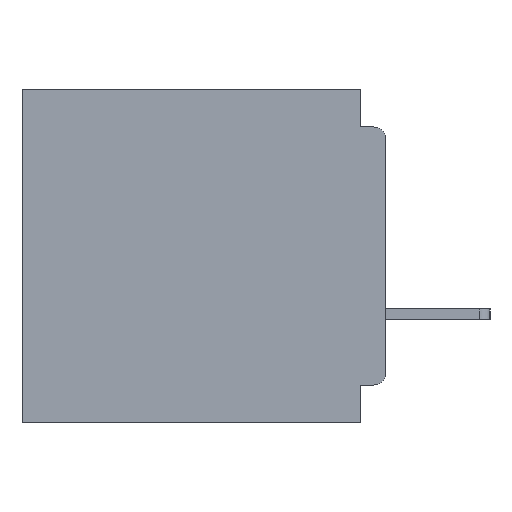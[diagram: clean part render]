
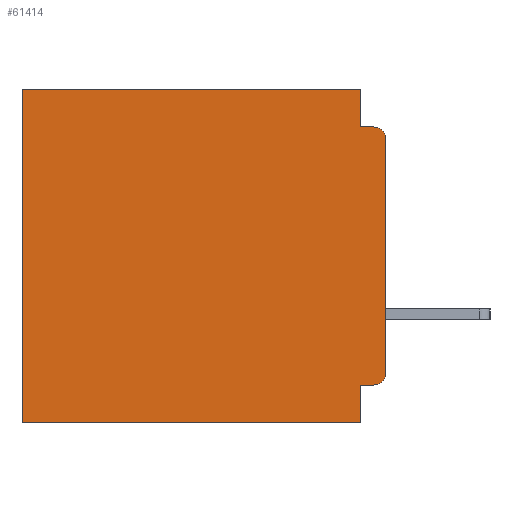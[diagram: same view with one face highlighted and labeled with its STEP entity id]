
A CAD part, left-side view. The second image highlights one B-rep face of the part: STEP entity #61414.
In plain terms, the highlighted planar face has unit normal (-1, 0, 0).
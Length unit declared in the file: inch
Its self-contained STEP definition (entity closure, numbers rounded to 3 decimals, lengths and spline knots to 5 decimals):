
#351 = CARTESIAN_POINT ( 'NONE',  ( 0.3, 0.437, 0. ) ) ;
#916 = ORIENTED_EDGE ( 'NONE', *, *, #24762, .F. ) ;
#1040 = CARTESIAN_POINT ( 'NONE',  ( 0.3, 0.031, -0.355 ) ) ;
#2915 = CARTESIAN_POINT ( 'NONE',  ( 0.3, 0.031, -0.4 ) ) ;
#5442 = CARTESIAN_POINT ( 'NONE',  ( 0.3, 0.015, -0.355 ) ) ;
#6471 = VECTOR ( 'NONE', #7966, 39.37008 ) ;
#6531 = EDGE_CURVE ( 'NONE', #40955, #40975, #32514, .T. ) ;
#6659 = VECTOR ( 'NONE', #20044, 39.37008 ) ;
#7397 = CARTESIAN_POINT ( 'NONE',  ( 0.3, 0., -0.34 ) ) ;
#7966 = DIRECTION ( 'NONE',  ( 0., 0., -1. ) ) ;
#9464 = AXIS2_PLACEMENT_3D ( 'NONE', #40787, #11779, #45653 ) ;
#9572 = DIRECTION ( 'NONE',  ( 0., 0., -1. ) ) ;
#9650 = CARTESIAN_POINT ( 'NONE',  ( 0.3, 0.015, -0.34 ) ) ;
#9901 = VECTOR ( 'NONE', #31762, 39.37008 ) ;
#9990 = VECTOR ( 'NONE', #12274, 39.37008 ) ;
#11779 = DIRECTION ( 'NONE',  ( -1., 0., 0. ) ) ;
#12274 = DIRECTION ( 'NONE',  ( 0., -1., 0. ) ) ;
#12869 = CARTESIAN_POINT ( 'NONE',  ( 0.3, 0.031, -0.4 ) ) ;
#13371 = EDGE_CURVE ( 'NONE', #30575, #21173, #24638, .T. ) ;
#13709 = DIRECTION ( 'NONE',  ( 0., 1., 0. ) ) ;
#13722 = VERTEX_POINT ( 'NONE', #39696 ) ;
#14562 = DIRECTION ( 'NONE',  ( 0., 0., -1. ) ) ;
#14825 = DIRECTION ( 'NONE',  ( 1., 0., 0. ) ) ;
#15060 = EDGE_CURVE ( 'NONE', #29861, #50919, #62801, .T. ) ;
#16568 = ORIENTED_EDGE ( 'NONE', *, *, #6531, .F. ) ;
#17241 = AXIS2_PLACEMENT_3D ( 'NONE', #9650, #43543, #14562 ) ;
#18829 = VECTOR ( 'NONE', #9572, 39.37008 ) ;
#19095 = EDGE_CURVE ( 'NONE', #25048, #40975, #49590, .T. ) ;
#20044 = DIRECTION ( 'NONE',  ( 0., 0., -1. ) ) ;
#20284 = ORIENTED_EDGE ( 'NONE', *, *, #28108, .T. ) ;
#21173 = VERTEX_POINT ( 'NONE', #45372 ) ;
#22085 = CARTESIAN_POINT ( 'NONE',  ( 0.3, 0., 0. ) ) ;
#22993 = LINE ( 'NONE', #50999, #9990 ) ;
#23449 = EDGE_LOOP ( 'NONE', ( #16568, #20284, #916, #38495, #24552, #29394, #49264, #24599, #29490, #45319 ) ) ;
#23520 = CARTESIAN_POINT ( 'NONE',  ( 0.3, 0., -0.355 ) ) ;
#24063 = CARTESIAN_POINT ( 'NONE',  ( 0.3, 0.031, 0. ) ) ;
#24552 = ORIENTED_EDGE ( 'NONE', *, *, #15060, .T. ) ;
#24599 = ORIENTED_EDGE ( 'NONE', *, *, #59962, .F. ) ;
#24638 = LINE ( 'NONE', #34206, #48790 ) ;
#24762 = EDGE_CURVE ( 'NONE', #57571, #13722, #22993, .T. ) ;
#25048 = VERTEX_POINT ( 'NONE', #5442 ) ;
#25126 = CARTESIAN_POINT ( 'NONE',  ( 0.3, 0., -0.4 ) ) ;
#26385 = VECTOR ( 'NONE', #13709, 39.37008 ) ;
#27464 = EDGE_CURVE ( 'NONE', #25048, #47834, #27925, .T. ) ;
#27925 = LINE ( 'NONE', #23520, #26385 ) ;
#28108 = EDGE_CURVE ( 'NONE', #40955, #13722, #39850, .T. ) ;
#29210 = DIRECTION ( 'NONE',  ( 0., 1., 0. ) ) ;
#29394 = ORIENTED_EDGE ( 'NONE', *, *, #47730, .T. ) ;
#29490 = ORIENTED_EDGE ( 'NONE', *, *, #27464, .F. ) ;
#29861 = VERTEX_POINT ( 'NONE', #41222 ) ;
#30575 = VERTEX_POINT ( 'NONE', #2915 ) ;
#31762 = DIRECTION ( 'NONE',  ( 0., 1., 0. ) ) ;
#32514 = LINE ( 'NONE', #25126, #6659 ) ;
#34206 = CARTESIAN_POINT ( 'NONE',  ( 0.3, 0., -0.4 ) ) ;
#35443 = CARTESIAN_POINT ( 'NONE',  ( 0.3, 0.031, -0.045 ) ) ;
#38495 = ORIENTED_EDGE ( 'NONE', *, *, #46556, .F. ) ;
#38903 = PLANE ( 'NONE',  #59714 ) ;
#39696 = CARTESIAN_POINT ( 'NONE',  ( 0.3, 0.015, -0.045 ) ) ;
#39850 = CIRCLE ( 'NONE', #9464, 0.015 ) ;
#40607 = LINE ( 'NONE', #12869, #6471 ) ;
#40787 = CARTESIAN_POINT ( 'NONE',  ( 0.3, 0.015, -0.06 ) ) ;
#40955 = VERTEX_POINT ( 'NONE', #50817 ) ;
#40975 = VERTEX_POINT ( 'NONE', #7397 ) ;
#41222 = CARTESIAN_POINT ( 'NONE',  ( 0.3, 0.031, 0. ) ) ;
#43543 = DIRECTION ( 'NONE',  ( -1., 0., 0. ) ) ;
#43793 = CARTESIAN_POINT ( 'NONE',  ( 0.3, 0., -0.4 ) ) ;
#44497 = LINE ( 'NONE', #24063, #18829 ) ;
#45319 = ORIENTED_EDGE ( 'NONE', *, *, #19095, .T. ) ;
#45372 = CARTESIAN_POINT ( 'NONE',  ( 0.3, 0.437, -0.4 ) ) ;
#45653 = DIRECTION ( 'NONE',  ( 0., 0., -1. ) ) ;
#46224 = FACE_OUTER_BOUND ( 'NONE', #23449, .T. ) ;
#46556 = EDGE_CURVE ( 'NONE', #29861, #57571, #44497, .T. ) ;
#47354 = VECTOR ( 'NONE', #58229, 39.37008 ) ;
#47730 = EDGE_CURVE ( 'NONE', #50919, #21173, #50383, .T. ) ;
#47834 = VERTEX_POINT ( 'NONE', #1040 ) ;
#48657 = DIRECTION ( 'NONE',  ( 0., 0., -1. ) ) ;
#48790 = VECTOR ( 'NONE', #29210, 39.37008 ) ;
#49264 = ORIENTED_EDGE ( 'NONE', *, *, #13371, .F. ) ;
#49590 = CIRCLE ( 'NONE', #17241, 0.015 ) ;
#50383 = LINE ( 'NONE', #53401, #47354 ) ;
#50817 = CARTESIAN_POINT ( 'NONE',  ( 0.3, 0., -0.06 ) ) ;
#50919 = VERTEX_POINT ( 'NONE', #351 ) ;
#50999 = CARTESIAN_POINT ( 'NONE',  ( 0.3, 0., -0.045 ) ) ;
#53401 = CARTESIAN_POINT ( 'NONE',  ( 0.3, 0.437, -0.4 ) ) ;
#57571 = VERTEX_POINT ( 'NONE', #35443 ) ;
#58229 = DIRECTION ( 'NONE',  ( 0., 0., -1. ) ) ;
#59714 = AXIS2_PLACEMENT_3D ( 'NONE', #43793, #14825, #48657 ) ;
#59962 = EDGE_CURVE ( 'NONE', #47834, #30575, #40607, .T. ) ;
#61414 = ADVANCED_FACE ( 'NONE', ( #46224 ), #38903, .F. ) ;
#62801 = LINE ( 'NONE', #22085, #9901 ) ;
